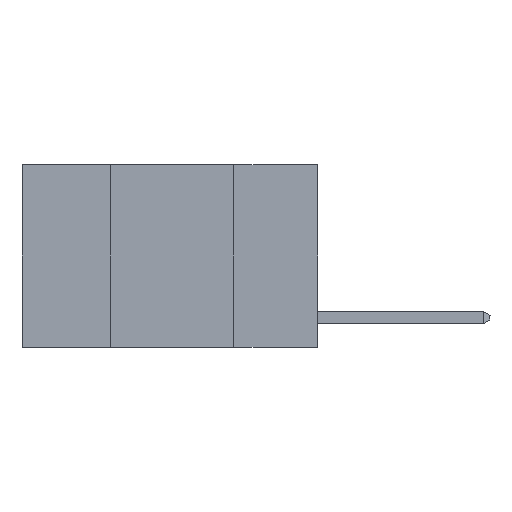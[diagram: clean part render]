
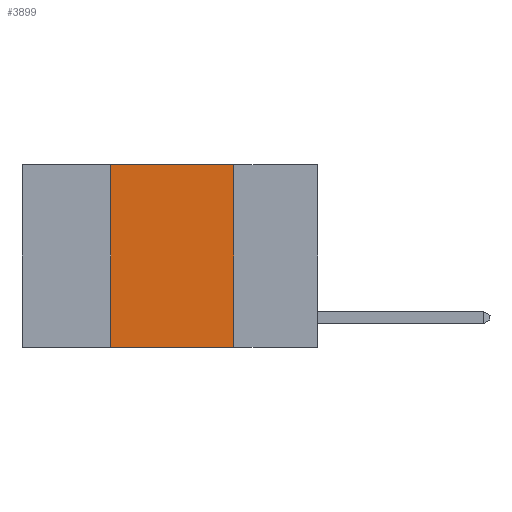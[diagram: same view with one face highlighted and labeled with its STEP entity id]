
A CAD part, left-side view. The second image highlights one B-rep face of the part: STEP entity #3899.
In plain terms, the highlighted planar face has unit normal (-1, 0, 0).
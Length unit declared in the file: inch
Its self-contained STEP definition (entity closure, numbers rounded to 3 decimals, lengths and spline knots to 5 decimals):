
#197 = CARTESIAN_POINT ( 'NONE',  ( 0., 0.17, 0. ) ) ;
#786 = PLANE ( 'NONE',  #9611 ) ;
#889 = CARTESIAN_POINT ( 'NONE',  ( 0., 0.42, -0.37 ) ) ;
#969 = EDGE_CURVE ( 'NONE', #5311, #2301, #7225, .T. ) ;
#1269 = ORIENTED_EDGE ( 'NONE', *, *, #969, .F. ) ;
#1314 = DIRECTION ( 'NONE',  ( 0., 0., -1. ) ) ;
#2301 = VERTEX_POINT ( 'NONE', #197 ) ;
#2419 = CARTESIAN_POINT ( 'NONE',  ( 0., 0.17, -0.37 ) ) ;
#2770 = CARTESIAN_POINT ( 'NONE',  ( 0., 0.6, 0. ) ) ;
#3053 = VECTOR ( 'NONE', #7850, 39.37008 ) ;
#3478 = ORIENTED_EDGE ( 'NONE', *, *, #5298, .F. ) ;
#3514 = LINE ( 'NONE', #6351, #5334 ) ;
#3732 = LINE ( 'NONE', #13141, #5073 ) ;
#3899 = ADVANCED_FACE ( 'NONE', ( #12818 ), #786, .F. ) ;
#4652 = VERTEX_POINT ( 'NONE', #2419 ) ;
#4688 = DIRECTION ( 'NONE',  ( 0., 0., 1. ) ) ;
#5073 = VECTOR ( 'NONE', #4688, 39.37008 ) ;
#5298 = EDGE_CURVE ( 'NONE', #11932, #5311, #3732, .T. ) ;
#5311 = VERTEX_POINT ( 'NONE', #6832 ) ;
#5334 = VECTOR ( 'NONE', #6210, 39.37008 ) ;
#6210 = DIRECTION ( 'NONE',  ( 0., -1., 0. ) ) ;
#6351 = CARTESIAN_POINT ( 'NONE',  ( 0., 0.6, -0.37 ) ) ;
#6832 = CARTESIAN_POINT ( 'NONE',  ( 0., 0.42, 0. ) ) ;
#6843 = EDGE_CURVE ( 'NONE', #2301, #4652, #7443, .T. ) ;
#7225 = LINE ( 'NONE', #12173, #3053 ) ;
#7443 = LINE ( 'NONE', #11898, #8447 ) ;
#7850 = DIRECTION ( 'NONE',  ( 0., -1., 0. ) ) ;
#8447 = VECTOR ( 'NONE', #1314, 39.37008 ) ;
#9611 = AXIS2_PLACEMENT_3D ( 'NONE', #2770, #13453, #12485 ) ;
#10060 = EDGE_CURVE ( 'NONE', #11932, #4652, #3514, .T. ) ;
#11823 = ORIENTED_EDGE ( 'NONE', *, *, #6843, .F. ) ;
#11898 = CARTESIAN_POINT ( 'NONE',  ( 0., 0.17, 0. ) ) ;
#11930 = ORIENTED_EDGE ( 'NONE', *, *, #10060, .T. ) ;
#11932 = VERTEX_POINT ( 'NONE', #889 ) ;
#12173 = CARTESIAN_POINT ( 'NONE',  ( 0., 0.6, 0. ) ) ;
#12485 = DIRECTION ( 'NONE',  ( 0., 0., -1. ) ) ;
#12596 = EDGE_LOOP ( 'NONE', ( #11823, #1269, #3478, #11930 ) ) ;
#12818 = FACE_OUTER_BOUND ( 'NONE', #12596, .T. ) ;
#13141 = CARTESIAN_POINT ( 'NONE',  ( 0., 0.42, 0. ) ) ;
#13453 = DIRECTION ( 'NONE',  ( 1., 0., 0. ) ) ;
